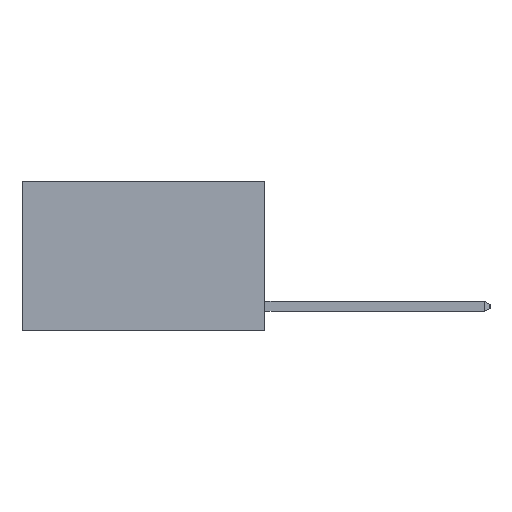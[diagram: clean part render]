
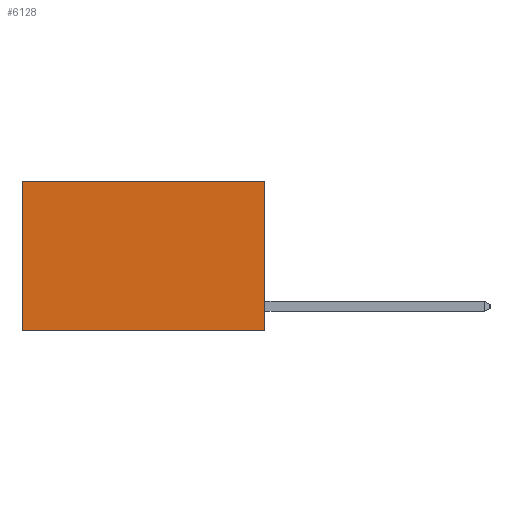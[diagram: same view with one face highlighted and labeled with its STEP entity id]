
A CAD part, left-side view. The second image highlights one B-rep face of the part: STEP entity #6128.
In plain terms, the highlighted planar face has unit normal (-1, 0, 0).
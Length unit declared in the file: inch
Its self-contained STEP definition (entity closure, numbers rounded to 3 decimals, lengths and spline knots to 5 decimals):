
#128 = DIRECTION ( 'NONE',  ( 1., 0., 0. ) ) ;
#306 = EDGE_CURVE ( 'NONE', #6853, #6250, #4940, .T. ) ;
#772 = EDGE_LOOP ( 'NONE', ( #6914, #6741, #6929, #6967 ) ) ;
#958 = CARTESIAN_POINT ( 'NONE',  ( 0.2625, 0.6, -0.37 ) ) ;
#1013 = FACE_OUTER_BOUND ( 'NONE', #772, .T. ) ;
#1235 = DIRECTION ( 'NONE',  ( 0., 1., 0. ) ) ;
#1361 = CARTESIAN_POINT ( 'NONE',  ( 0.2625, 0., 0. ) ) ;
#1409 = VECTOR ( 'NONE', #6556, 39.37008 ) ;
#1477 = PLANE ( 'NONE',  #3128 ) ;
#1757 = VECTOR ( 'NONE', #1235, 39.37008 ) ;
#1926 = EDGE_CURVE ( 'NONE', #2460, #6250, #7072, .T. ) ;
#2277 = VECTOR ( 'NONE', #7255, 39.37008 ) ;
#2460 = VERTEX_POINT ( 'NONE', #6730 ) ;
#3075 = CARTESIAN_POINT ( 'NONE',  ( 0.2625, 0., 0. ) ) ;
#3128 = AXIS2_PLACEMENT_3D ( 'NONE', #6808, #128, #4531 ) ;
#3522 = EDGE_CURVE ( 'NONE', #5988, #6853, #5243, .T. ) ;
#4531 = DIRECTION ( 'NONE',  ( 0., 0., -1. ) ) ;
#4940 = LINE ( 'NONE', #6583, #1757 ) ;
#5243 = LINE ( 'NONE', #1361, #2277 ) ;
#5363 = CARTESIAN_POINT ( 'NONE',  ( 0.2625, 0., -0.37 ) ) ;
#5988 = VERTEX_POINT ( 'NONE', #6103 ) ;
#6103 = CARTESIAN_POINT ( 'NONE',  ( 0.2625, 0., 0. ) ) ;
#6128 = ADVANCED_FACE ( 'NONE', ( #1013 ), #1477, .F. ) ;
#6250 = VERTEX_POINT ( 'NONE', #958 ) ;
#6324 = LINE ( 'NONE', #3075, #1409 ) ;
#6556 = DIRECTION ( 'NONE',  ( 0., 1., 0. ) ) ;
#6583 = CARTESIAN_POINT ( 'NONE',  ( 0.2625, 0., -0.37 ) ) ;
#6730 = CARTESIAN_POINT ( 'NONE',  ( 0.2625, 0.6, 0. ) ) ;
#6741 = ORIENTED_EDGE ( 'NONE', *, *, #306, .F. ) ;
#6808 = CARTESIAN_POINT ( 'NONE',  ( 0.2625, 0., 0. ) ) ;
#6853 = VERTEX_POINT ( 'NONE', #5363 ) ;
#6885 = VECTOR ( 'NONE', #7090, 39.37008 ) ;
#6914 = ORIENTED_EDGE ( 'NONE', *, *, #1926, .T. ) ;
#6915 = EDGE_CURVE ( 'NONE', #5988, #2460, #6324, .T. ) ;
#6929 = ORIENTED_EDGE ( 'NONE', *, *, #3522, .F. ) ;
#6967 = ORIENTED_EDGE ( 'NONE', *, *, #6915, .T. ) ;
#7072 = LINE ( 'NONE', #7384, #6885 ) ;
#7090 = DIRECTION ( 'NONE',  ( 0., 0., -1. ) ) ;
#7255 = DIRECTION ( 'NONE',  ( 0., 0., -1. ) ) ;
#7384 = CARTESIAN_POINT ( 'NONE',  ( 0.2625, 0.6, 0. ) ) ;
